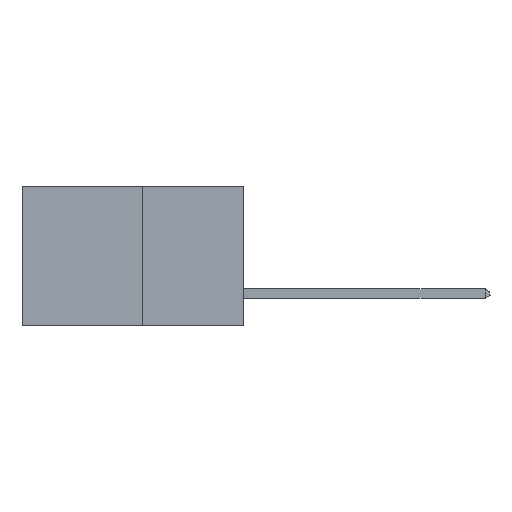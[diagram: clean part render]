
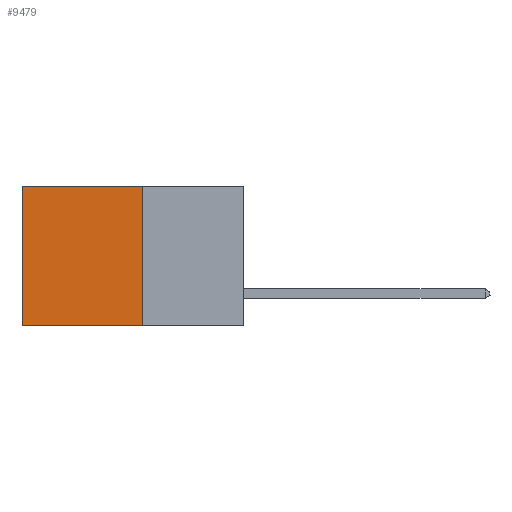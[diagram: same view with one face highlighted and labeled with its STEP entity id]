
A CAD part, left-side view. The second image highlights one B-rep face of the part: STEP entity #9479.
In plain terms, the highlighted planar face has unit normal (-1, 0, 0).
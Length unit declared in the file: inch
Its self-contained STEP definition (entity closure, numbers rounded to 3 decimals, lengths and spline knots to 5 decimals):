
#197 = ORIENTED_EDGE ( 'NONE', *, *, #4070, .T. ) ;
#712 = VECTOR ( 'NONE', #14219, 39.37008 ) ;
#749 = EDGE_CURVE ( 'NONE', #5280, #4808, #1119, .T. ) ;
#802 = CARTESIAN_POINT ( 'NONE',  ( 0.277, 0.27, -0.37 ) ) ;
#1119 = LINE ( 'NONE', #6932, #712 ) ;
#1502 = VECTOR ( 'NONE', #15290, 39.37008 ) ;
#1921 = LINE ( 'NONE', #11758, #1502 ) ;
#2413 = EDGE_LOOP ( 'NONE', ( #13472, #7991, #13462, #197 ) ) ;
#2636 = DIRECTION ( 'NONE',  ( 0., 0., -1. ) ) ;
#2910 = VERTEX_POINT ( 'NONE', #4123 ) ;
#3742 = DIRECTION ( 'NONE',  ( 0., 1., 0. ) ) ;
#3827 = CARTESIAN_POINT ( 'NONE',  ( 0.277, 0.59, -0.37 ) ) ;
#4070 = EDGE_CURVE ( 'NONE', #10074, #2910, #7233, .T. ) ;
#4123 = CARTESIAN_POINT ( 'NONE',  ( 0.277, 0.59, 0. ) ) ;
#4387 = VECTOR ( 'NONE', #3742, 39.37008 ) ;
#4808 = VERTEX_POINT ( 'NONE', #3827 ) ;
#5280 = VERTEX_POINT ( 'NONE', #13209 ) ;
#6932 = CARTESIAN_POINT ( 'NONE',  ( 0.277, 0.27, -0.37 ) ) ;
#7163 = DIRECTION ( 'NONE',  ( 1., 0., 0. ) ) ;
#7233 = LINE ( 'NONE', #10887, #4387 ) ;
#7968 = EDGE_CURVE ( 'NONE', #10074, #5280, #11480, .T. ) ;
#7991 = ORIENTED_EDGE ( 'NONE', *, *, #749, .F. ) ;
#9479 = ADVANCED_FACE ( 'NONE', ( #14027 ), #14150, .F. ) ;
#9894 = CARTESIAN_POINT ( 'NONE',  ( 0.277, 0.27, -0.37 ) ) ;
#10074 = VERTEX_POINT ( 'NONE', #10748 ) ;
#10748 = CARTESIAN_POINT ( 'NONE',  ( 0.277, 0.27, 0. ) ) ;
#10887 = CARTESIAN_POINT ( 'NONE',  ( 0.277, 0.27, 0. ) ) ;
#11480 = LINE ( 'NONE', #9894, #14622 ) ;
#11758 = CARTESIAN_POINT ( 'NONE',  ( 0.277, 0.59, -0.37 ) ) ;
#11942 = EDGE_CURVE ( 'NONE', #2910, #4808, #1921, .T. ) ;
#13209 = CARTESIAN_POINT ( 'NONE',  ( 0.277, 0.27, -0.37 ) ) ;
#13462 = ORIENTED_EDGE ( 'NONE', *, *, #7968, .F. ) ;
#13472 = ORIENTED_EDGE ( 'NONE', *, *, #11942, .T. ) ;
#14027 = FACE_OUTER_BOUND ( 'NONE', #2413, .T. ) ;
#14150 = PLANE ( 'NONE',  #14926 ) ;
#14219 = DIRECTION ( 'NONE',  ( 0., 1., 0. ) ) ;
#14622 = VECTOR ( 'NONE', #2636, 39.37008 ) ;
#14926 = AXIS2_PLACEMENT_3D ( 'NONE', #802, #7163, #15306 ) ;
#15290 = DIRECTION ( 'NONE',  ( 0., 0., -1. ) ) ;
#15306 = DIRECTION ( 'NONE',  ( 0., 0., -1. ) ) ;
